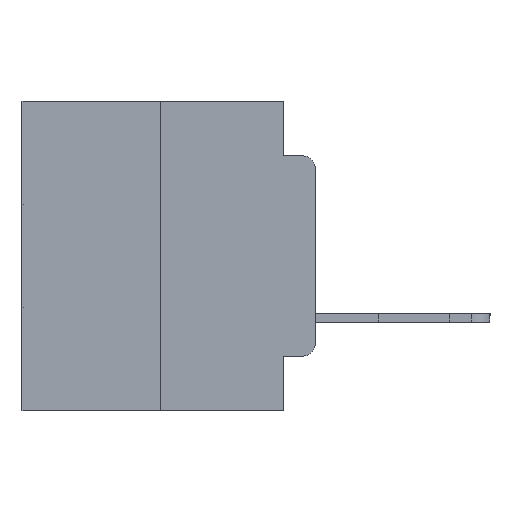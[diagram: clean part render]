
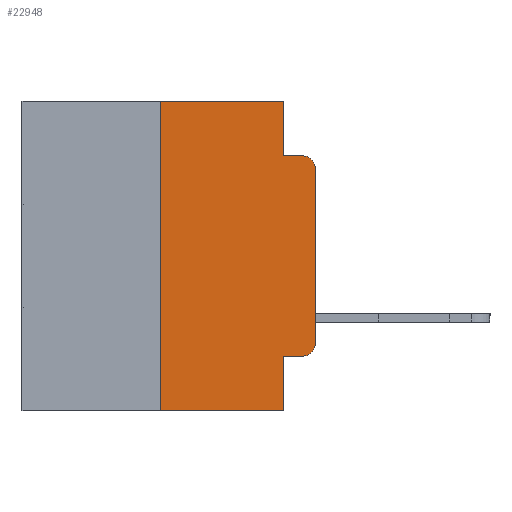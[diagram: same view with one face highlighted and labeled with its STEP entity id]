
A CAD part, left-side view. The second image highlights one B-rep face of the part: STEP entity #22948.
In plain terms, the highlighted planar face has unit normal (-1, 0, 0).
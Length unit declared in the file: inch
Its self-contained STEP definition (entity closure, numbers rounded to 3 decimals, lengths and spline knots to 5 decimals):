
#692 = DIRECTION ( 'NONE',  ( 0., 0., 1. ) ) ;
#795 = EDGE_CURVE ( 'NONE', #16612, #7098, #16607, .T. ) ;
#935 = CARTESIAN_POINT ( 'NONE',  ( 0., 0., 0. ) ) ;
#980 = LINE ( 'NONE', #17105, #11426 ) ;
#1274 = CARTESIAN_POINT ( 'NONE',  ( 0., 0.051, 0. ) ) ;
#1377 = CARTESIAN_POINT ( 'NONE',  ( 0., 0.25, 0. ) ) ;
#1569 = AXIS2_PLACEMENT_3D ( 'NONE', #20587, #24654, #12449 ) ;
#2167 = EDGE_CURVE ( 'NONE', #25141, #7098, #8201, .T. ) ;
#2425 = CARTESIAN_POINT ( 'NONE',  ( 0., 0.051, -0.4115 ) ) ;
#3052 = ORIENTED_EDGE ( 'NONE', *, *, #15214, .T. ) ;
#3237 = AXIS2_PLACEMENT_3D ( 'NONE', #7815, #22176, #9926 ) ;
#3518 = EDGE_CURVE ( 'NONE', #12951, #25141, #4795, .T. ) ;
#3793 = CIRCLE ( 'NONE', #3237, 0.02 ) ;
#3863 = LINE ( 'NONE', #25997, #14952 ) ;
#4055 = EDGE_LOOP ( 'NONE', ( #18564, #23999, #13797, #25271, #9637, #5334, #16377, #17600, #7992, #3052 ) ) ;
#4795 = LINE ( 'NONE', #935, #15219 ) ;
#4890 = DIRECTION ( 'NONE',  ( 0., 0., 1. ) ) ;
#5334 = ORIENTED_EDGE ( 'NONE', *, *, #22047, .F. ) ;
#5650 = AXIS2_PLACEMENT_3D ( 'NONE', #16119, #6917, #15447 ) ;
#5830 = LINE ( 'NONE', #10519, #10782 ) ;
#6917 = DIRECTION ( 'NONE',  ( -1., 0., 0. ) ) ;
#7098 = VERTEX_POINT ( 'NONE', #15718 ) ;
#7304 = LINE ( 'NONE', #2425, #12846 ) ;
#7644 = DIRECTION ( 'NONE',  ( 0., -1., 0. ) ) ;
#7815 = CARTESIAN_POINT ( 'NONE',  ( 0., 0.02, -0.3915 ) ) ;
#7992 = ORIENTED_EDGE ( 'NONE', *, *, #16575, .T. ) ;
#8172 = CARTESIAN_POINT ( 'NONE',  ( 0., 0.25, -0.5 ) ) ;
#8201 = CIRCLE ( 'NONE', #5650, 0.02 ) ;
#8524 = VERTEX_POINT ( 'NONE', #8172 ) ;
#9265 = VERTEX_POINT ( 'NONE', #20775 ) ;
#9284 = FACE_OUTER_BOUND ( 'NONE', #4055, .T. ) ;
#9386 = EDGE_CURVE ( 'NONE', #8524, #11990, #980, .T. ) ;
#9637 = ORIENTED_EDGE ( 'NONE', *, *, #19316, .F. ) ;
#9926 = DIRECTION ( 'NONE',  ( 0., 0., -1. ) ) ;
#10519 = CARTESIAN_POINT ( 'NONE',  ( 0., 0.051, 0. ) ) ;
#10635 = VERTEX_POINT ( 'NONE', #18972 ) ;
#10782 = VECTOR ( 'NONE', #16661, 39.37008 ) ;
#10793 = LINE ( 'NONE', #1274, #15581 ) ;
#11109 = CARTESIAN_POINT ( 'NONE',  ( 0., 0.25, 0. ) ) ;
#11300 = VECTOR ( 'NONE', #692, 39.37008 ) ;
#11426 = VECTOR ( 'NONE', #19126, 39.37008 ) ;
#11990 = VERTEX_POINT ( 'NONE', #19535 ) ;
#12449 = DIRECTION ( 'NONE',  ( 0., 0., -1. ) ) ;
#12846 = VECTOR ( 'NONE', #16923, 39.37008 ) ;
#12951 = VERTEX_POINT ( 'NONE', #24059 ) ;
#13717 = DIRECTION ( 'NONE',  ( 0., 0., -1. ) ) ;
#13797 = ORIENTED_EDGE ( 'NONE', *, *, #795, .F. ) ;
#14522 = VERTEX_POINT ( 'NONE', #25311 ) ;
#14713 = VERTEX_POINT ( 'NONE', #1377 ) ;
#14952 = VECTOR ( 'NONE', #7644, 39.37008 ) ;
#15214 = EDGE_CURVE ( 'NONE', #14522, #12951, #3793, .T. ) ;
#15219 = VECTOR ( 'NONE', #4890, 39.37008 ) ;
#15447 = DIRECTION ( 'NONE',  ( 0., 0., -1. ) ) ;
#15581 = VECTOR ( 'NONE', #13717, 39.37008 ) ;
#15718 = CARTESIAN_POINT ( 'NONE',  ( 0., 0.02, -0.0885 ) ) ;
#16119 = CARTESIAN_POINT ( 'NONE',  ( 0., 0.02, -0.1085 ) ) ;
#16377 = ORIENTED_EDGE ( 'NONE', *, *, #9386, .T. ) ;
#16485 = PLANE ( 'NONE',  #1569 ) ;
#16575 = EDGE_CURVE ( 'NONE', #9265, #14522, #7304, .T. ) ;
#16607 = LINE ( 'NONE', #18991, #20755 ) ;
#16612 = VERTEX_POINT ( 'NONE', #17003 ) ;
#16661 = DIRECTION ( 'NONE',  ( 0., 0., -1. ) ) ;
#16923 = DIRECTION ( 'NONE',  ( 0., -1., 0. ) ) ;
#17003 = CARTESIAN_POINT ( 'NONE',  ( 0., 0.051, -0.0885 ) ) ;
#17105 = CARTESIAN_POINT ( 'NONE',  ( 0., 0.473, -0.5 ) ) ;
#17342 = LINE ( 'NONE', #11109, #11300 ) ;
#17600 = ORIENTED_EDGE ( 'NONE', *, *, #19276, .F. ) ;
#18564 = ORIENTED_EDGE ( 'NONE', *, *, #3518, .T. ) ;
#18972 = CARTESIAN_POINT ( 'NONE',  ( 0., 0.051, 0. ) ) ;
#18991 = CARTESIAN_POINT ( 'NONE',  ( 0., 0.051, -0.0885 ) ) ;
#19126 = DIRECTION ( 'NONE',  ( 0., -1., 0. ) ) ;
#19276 = EDGE_CURVE ( 'NONE', #9265, #11990, #10793, .T. ) ;
#19316 = EDGE_CURVE ( 'NONE', #14713, #10635, #3863, .T. ) ;
#19535 = CARTESIAN_POINT ( 'NONE',  ( 0., 0.051, -0.5 ) ) ;
#20587 = CARTESIAN_POINT ( 'NONE',  ( 0., 0.473, 0. ) ) ;
#20755 = VECTOR ( 'NONE', #21573, 39.37008 ) ;
#20775 = CARTESIAN_POINT ( 'NONE',  ( 0., 0.051, -0.4115 ) ) ;
#21573 = DIRECTION ( 'NONE',  ( 0., -1., 0. ) ) ;
#22047 = EDGE_CURVE ( 'NONE', #8524, #14713, #17342, .T. ) ;
#22176 = DIRECTION ( 'NONE',  ( -1., 0., 0. ) ) ;
#22948 = ADVANCED_FACE ( 'NONE', ( #9284 ), #16485, .F. ) ;
#23398 = CARTESIAN_POINT ( 'NONE',  ( 0., 0., -0.1085 ) ) ;
#23999 = ORIENTED_EDGE ( 'NONE', *, *, #2167, .T. ) ;
#24059 = CARTESIAN_POINT ( 'NONE',  ( 0., 0., -0.3915 ) ) ;
#24654 = DIRECTION ( 'NONE',  ( 1., 0., 0. ) ) ;
#25141 = VERTEX_POINT ( 'NONE', #23398 ) ;
#25271 = ORIENTED_EDGE ( 'NONE', *, *, #26111, .F. ) ;
#25311 = CARTESIAN_POINT ( 'NONE',  ( 0., 0.02, -0.4115 ) ) ;
#25997 = CARTESIAN_POINT ( 'NONE',  ( 0., 0.473, 0. ) ) ;
#26111 = EDGE_CURVE ( 'NONE', #10635, #16612, #5830, .T. ) ;
